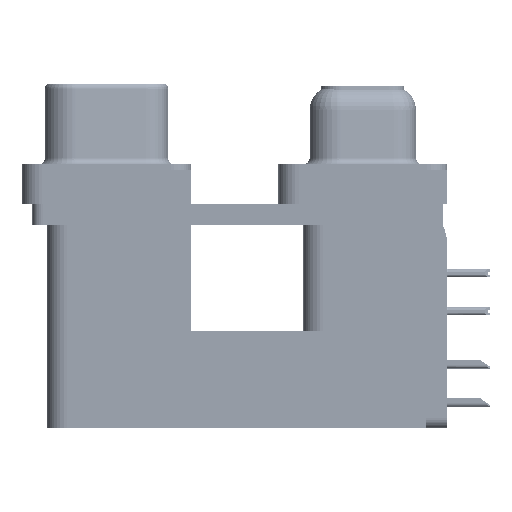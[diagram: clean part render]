
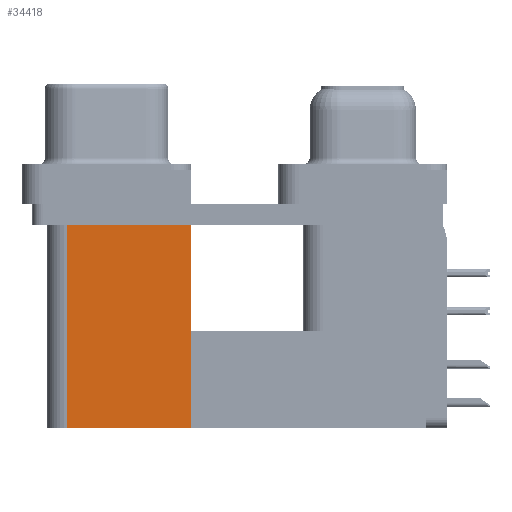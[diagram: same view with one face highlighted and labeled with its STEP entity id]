
A CAD part, left-side view. The second image highlights one B-rep face of the part: STEP entity #34418.
In plain terms, the highlighted planar face has unit normal (-1, 0, 0).
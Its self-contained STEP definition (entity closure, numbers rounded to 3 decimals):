
#1010 = VERTEX_POINT ( 'NONE', #7420 ) ;
#3903 = VECTOR ( 'NONE', #33521, 1000. ) ;
#5434 = DIRECTION ( 'NONE',  ( 0., 0., 1. ) ) ;
#5811 = DIRECTION ( 'NONE',  ( 0., 1., 0. ) ) ;
#5874 = CARTESIAN_POINT ( 'NONE',  ( 3.79, 21.975, -19.2 ) ) ;
#6411 = VECTOR ( 'NONE', #5811, 1000. ) ;
#7420 = CARTESIAN_POINT ( 'NONE',  ( 3.79, 12.775, -2.5 ) ) ;
#10445 = CARTESIAN_POINT ( 'NONE',  ( 3.79, 12.775, -2.5 ) ) ;
#14870 = AXIS2_PLACEMENT_3D ( 'NONE', #60889, #56906, #36783 ) ;
#15390 = CARTESIAN_POINT ( 'NONE',  ( 3.79, 12.775, -19.2 ) ) ;
#17090 = VERTEX_POINT ( 'NONE', #34773 ) ;
#17371 = LINE ( 'NONE', #43749, #3903 ) ;
#20325 = LINE ( 'NONE', #15390, #58612 ) ;
#28162 = CARTESIAN_POINT ( 'NONE',  ( 3.79, 21.975, -2.5 ) ) ;
#31522 = PLANE ( 'NONE',  #14870 ) ;
#33521 = DIRECTION ( 'NONE',  ( 0., 0., 1. ) ) ;
#34418 = ADVANCED_FACE ( 'NONE', ( #46684 ), #31522, .F. ) ;
#34773 = CARTESIAN_POINT ( 'NONE',  ( 3.79, 12.775, -19.2 ) ) ;
#36783 = DIRECTION ( 'NONE',  ( 0., 1., 0. ) ) ;
#41218 = VERTEX_POINT ( 'NONE', #5874 ) ;
#41422 = ORIENTED_EDGE ( 'NONE', *, *, #51162, .T. ) ;
#41677 = EDGE_LOOP ( 'NONE', ( #41422, #41883, #41916, #43807 ) ) ;
#41883 = ORIENTED_EDGE ( 'NONE', *, *, #42873, .F. ) ;
#41916 = ORIENTED_EDGE ( 'NONE', *, *, #59469, .F. ) ;
#42873 = EDGE_CURVE ( 'NONE', #41218, #57627, #17371, .T. ) ;
#43749 = CARTESIAN_POINT ( 'NONE',  ( 3.79, 21.975, -19.2 ) ) ;
#43807 = ORIENTED_EDGE ( 'NONE', *, *, #43889, .T. ) ;
#43889 = EDGE_CURVE ( 'NONE', #17090, #1010, #20325, .T. ) ;
#46684 = FACE_OUTER_BOUND ( 'NONE', #41677, .T. ) ;
#46917 = DIRECTION ( 'NONE',  ( 0., 1., 0. ) ) ;
#51162 = EDGE_CURVE ( 'NONE', #1010, #57627, #59961, .T. ) ;
#54440 = VECTOR ( 'NONE', #46917, 1000. ) ;
#56906 = DIRECTION ( 'NONE',  ( 1., 0., 0. ) ) ;
#57468 = CARTESIAN_POINT ( 'NONE',  ( 3.79, 12.775, -19.2 ) ) ;
#57627 = VERTEX_POINT ( 'NONE', #28162 ) ;
#57785 = LINE ( 'NONE', #57468, #54440 ) ;
#58612 = VECTOR ( 'NONE', #5434, 1000. ) ;
#59469 = EDGE_CURVE ( 'NONE', #17090, #41218, #57785, .T. ) ;
#59961 = LINE ( 'NONE', #10445, #6411 ) ;
#60889 = CARTESIAN_POINT ( 'NONE',  ( 3.79, 12.775, -19.2 ) ) ;
